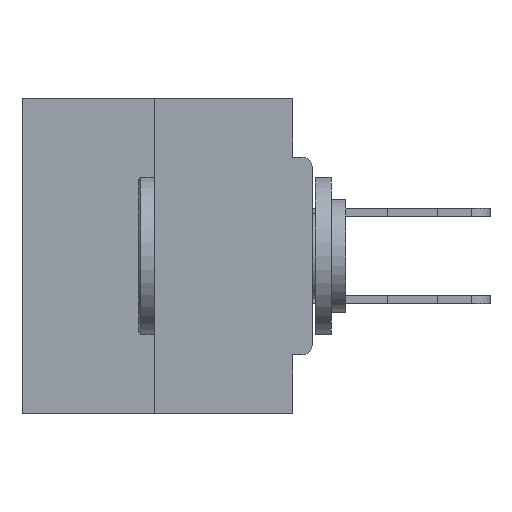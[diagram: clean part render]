
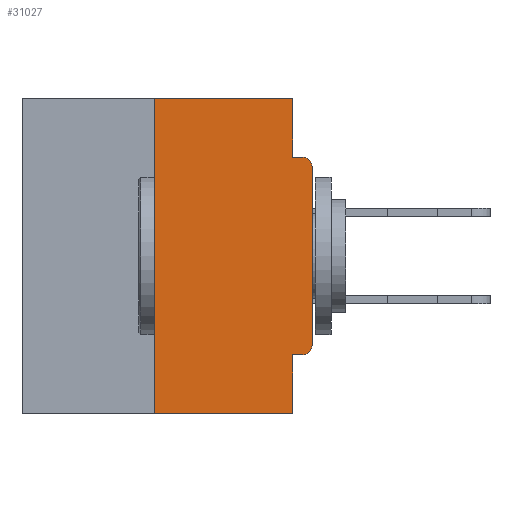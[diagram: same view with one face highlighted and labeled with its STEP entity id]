
A CAD part, left-side view. The second image highlights one B-rep face of the part: STEP entity #31027.
In plain terms, the highlighted planar face has unit normal (-1, 0, 0).
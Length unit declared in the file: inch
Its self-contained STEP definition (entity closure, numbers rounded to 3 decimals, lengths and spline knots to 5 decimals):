
#94 = ORIENTED_EDGE ( 'NONE', *, *, #28003, .T. ) ;
#652 = CIRCLE ( 'NONE', #5961, 0.015 ) ;
#1582 = VERTEX_POINT ( 'NONE', #3190 ) ;
#2150 = CARTESIAN_POINT ( 'NONE',  ( 0., 0.015, -0.1085 ) ) ;
#2363 = DIRECTION ( 'NONE',  ( 0., -1., 0. ) ) ;
#2643 = VECTOR ( 'NONE', #18528, 39.37008 ) ;
#2810 = CARTESIAN_POINT ( 'NONE',  ( 0., 0.46, 0. ) ) ;
#2912 = EDGE_CURVE ( 'NONE', #10054, #16567, #21278, .T. ) ;
#3170 = DIRECTION ( 'NONE',  ( 1., 0., 0. ) ) ;
#3190 = CARTESIAN_POINT ( 'NONE',  ( 0., 0.031, -0.4065 ) ) ;
#3434 = VECTOR ( 'NONE', #15646, 39.37008 ) ;
#3646 = VERTEX_POINT ( 'NONE', #20316 ) ;
#5570 = CARTESIAN_POINT ( 'NONE',  ( 0., 0.25, -0.5 ) ) ;
#5853 = EDGE_CURVE ( 'NONE', #10054, #24727, #11319, .T. ) ;
#5961 = AXIS2_PLACEMENT_3D ( 'NONE', #2150, #37600, #34522 ) ;
#6610 = PLANE ( 'NONE',  #35221 ) ;
#7821 = VERTEX_POINT ( 'NONE', #34718 ) ;
#8638 = CARTESIAN_POINT ( 'NONE',  ( 0., 0.031, 0. ) ) ;
#9346 = CIRCLE ( 'NONE', #18660, 0.015 ) ;
#9687 = ORIENTED_EDGE ( 'NONE', *, *, #28683, .F. ) ;
#9798 = VERTEX_POINT ( 'NONE', #29309 ) ;
#9871 = CARTESIAN_POINT ( 'NONE',  ( 0., 0.031, -0.5 ) ) ;
#10054 = VERTEX_POINT ( 'NONE', #5570 ) ;
#11319 = LINE ( 'NONE', #11936, #18206 ) ;
#11760 = EDGE_CURVE ( 'NONE', #7821, #32639, #11947, .T. ) ;
#11936 = CARTESIAN_POINT ( 'NONE',  ( 0., 0.25, 0. ) ) ;
#11947 = LINE ( 'NONE', #14824, #33504 ) ;
#12880 = ORIENTED_EDGE ( 'NONE', *, *, #5853, .F. ) ;
#13009 = ORIENTED_EDGE ( 'NONE', *, *, #16738, .T. ) ;
#14160 = VECTOR ( 'NONE', #2363, 39.37008 ) ;
#14824 = CARTESIAN_POINT ( 'NONE',  ( 0., 0., 0. ) ) ;
#15007 = CARTESIAN_POINT ( 'NONE',  ( 0., 0., -0.4065 ) ) ;
#15384 = LINE ( 'NONE', #2810, #18598 ) ;
#15464 = LINE ( 'NONE', #15578, #2643 ) ;
#15578 = CARTESIAN_POINT ( 'NONE',  ( 0., 0.031, 0. ) ) ;
#15646 = DIRECTION ( 'NONE',  ( 0., 0., -1. ) ) ;
#16004 = EDGE_CURVE ( 'NONE', #24727, #33235, #15384, .T. ) ;
#16567 = VERTEX_POINT ( 'NONE', #22578 ) ;
#16738 = EDGE_CURVE ( 'NONE', #3646, #7821, #9346, .T. ) ;
#16888 = ORIENTED_EDGE ( 'NONE', *, *, #16004, .F. ) ;
#17832 = VERTEX_POINT ( 'NONE', #29998 ) ;
#17994 = CARTESIAN_POINT ( 'NONE',  ( 0., 0., -0.0935 ) ) ;
#18206 = VECTOR ( 'NONE', #29388, 39.37008 ) ;
#18320 = CARTESIAN_POINT ( 'NONE',  ( 0., 0.46, -0.5 ) ) ;
#18499 = CARTESIAN_POINT ( 'NONE',  ( 0., 0.015, -0.3915 ) ) ;
#18528 = DIRECTION ( 'NONE',  ( 0., 0., -1. ) ) ;
#18598 = VECTOR ( 'NONE', #23023, 39.37008 ) ;
#18660 = AXIS2_PLACEMENT_3D ( 'NONE', #18499, #27087, #32983 ) ;
#18845 = EDGE_CURVE ( 'NONE', #1582, #16567, #35050, .T. ) ;
#20060 = ORIENTED_EDGE ( 'NONE', *, *, #2912, .T. ) ;
#20316 = CARTESIAN_POINT ( 'NONE',  ( 0., 0.015, -0.4065 ) ) ;
#20610 = LINE ( 'NONE', #15007, #34825 ) ;
#21278 = LINE ( 'NONE', #18320, #29989 ) ;
#22287 = EDGE_CURVE ( 'NONE', #33235, #9798, #15464, .T. ) ;
#22578 = CARTESIAN_POINT ( 'NONE',  ( 0., 0.031, -0.5 ) ) ;
#22866 = LINE ( 'NONE', #17994, #14160 ) ;
#23023 = DIRECTION ( 'NONE',  ( 0., -1., 0. ) ) ;
#24727 = VERTEX_POINT ( 'NONE', #26496 ) ;
#24834 = ORIENTED_EDGE ( 'NONE', *, *, #22287, .F. ) ;
#25012 = ORIENTED_EDGE ( 'NONE', *, *, #18845, .F. ) ;
#25057 = EDGE_CURVE ( 'NONE', #9798, #17832, #22866, .T. ) ;
#26472 = ORIENTED_EDGE ( 'NONE', *, *, #11760, .T. ) ;
#26496 = CARTESIAN_POINT ( 'NONE',  ( 0., 0.25, 0. ) ) ;
#27087 = DIRECTION ( 'NONE',  ( -1., 0., 0. ) ) ;
#28003 = EDGE_CURVE ( 'NONE', #32639, #17832, #652, .T. ) ;
#28683 = EDGE_CURVE ( 'NONE', #3646, #1582, #20610, .T. ) ;
#29207 = FACE_OUTER_BOUND ( 'NONE', #30847, .T. ) ;
#29309 = CARTESIAN_POINT ( 'NONE',  ( 0., 0.031, -0.0935 ) ) ;
#29388 = DIRECTION ( 'NONE',  ( 0., 0., 1. ) ) ;
#29672 = DIRECTION ( 'NONE',  ( 0., 0., -1. ) ) ;
#29708 = DIRECTION ( 'NONE',  ( 0., 0., 1. ) ) ;
#29989 = VECTOR ( 'NONE', #33064, 39.37008 ) ;
#29998 = CARTESIAN_POINT ( 'NONE',  ( 0., 0.015, -0.0935 ) ) ;
#30847 = EDGE_LOOP ( 'NONE', ( #16888, #12880, #20060, #25012, #9687, #13009, #26472, #94, #33987, #24834 ) ) ;
#31027 = ADVANCED_FACE ( 'NONE', ( #29207 ), #6610, .F. ) ;
#32639 = VERTEX_POINT ( 'NONE', #37913 ) ;
#32983 = DIRECTION ( 'NONE',  ( 0., 0., -1. ) ) ;
#33064 = DIRECTION ( 'NONE',  ( 0., -1., 0. ) ) ;
#33235 = VERTEX_POINT ( 'NONE', #8638 ) ;
#33504 = VECTOR ( 'NONE', #29708, 39.37008 ) ;
#33987 = ORIENTED_EDGE ( 'NONE', *, *, #25057, .F. ) ;
#34522 = DIRECTION ( 'NONE',  ( 0., 0., -1. ) ) ;
#34718 = CARTESIAN_POINT ( 'NONE',  ( 0., 0., -0.3915 ) ) ;
#34825 = VECTOR ( 'NONE', #35376, 39.37008 ) ;
#35050 = LINE ( 'NONE', #9871, #3434 ) ;
#35221 = AXIS2_PLACEMENT_3D ( 'NONE', #35291, #3170, #29672 ) ;
#35291 = CARTESIAN_POINT ( 'NONE',  ( 0., 0.46, 0. ) ) ;
#35376 = DIRECTION ( 'NONE',  ( 0., 1., 0. ) ) ;
#37600 = DIRECTION ( 'NONE',  ( -1., 0., 0. ) ) ;
#37913 = CARTESIAN_POINT ( 'NONE',  ( 0., 0., -0.1085 ) ) ;
